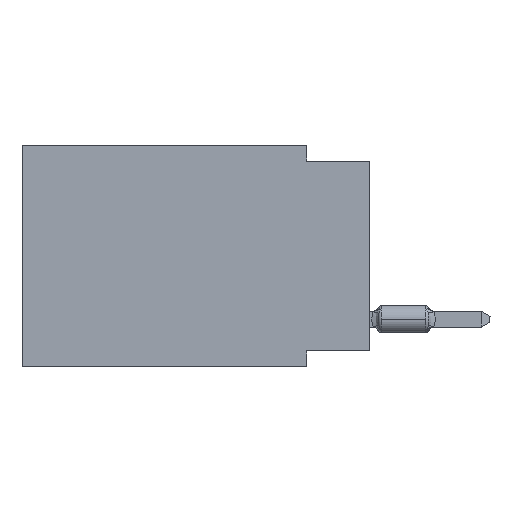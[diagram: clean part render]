
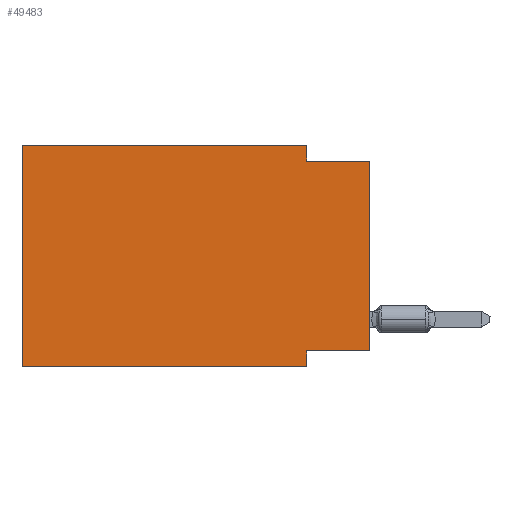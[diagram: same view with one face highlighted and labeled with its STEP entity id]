
A CAD part, left-side view. The second image highlights one B-rep face of the part: STEP entity #49483.
In plain terms, the highlighted planar face has unit normal (-1, 0, 0).
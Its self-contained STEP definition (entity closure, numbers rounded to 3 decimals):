
#1197 = CARTESIAN_POINT ( 'NONE',  ( 0., 2.54, -0.635 ) ) ;
#2183 = LINE ( 'NONE', #63998, #44489 ) ;
#3015 = VERTEX_POINT ( 'NONE', #1197 ) ;
#3428 = CARTESIAN_POINT ( 'NONE',  ( 0., 0., 0. ) ) ;
#4145 = EDGE_CURVE ( 'NONE', #8017, #71424, #2183, .T. ) ;
#4315 = LINE ( 'NONE', #15302, #61417 ) ;
#7125 = ORIENTED_EDGE ( 'NONE', *, *, #34295, .F. ) ;
#7843 = EDGE_CURVE ( 'NONE', #71424, #58549, #4315, .T. ) ;
#8017 = VERTEX_POINT ( 'NONE', #29485 ) ;
#8047 = DIRECTION ( 'NONE',  ( 0., 1., 0. ) ) ;
#8056 = AXIS2_PLACEMENT_3D ( 'NONE', #58355, #60075, #41530 ) ;
#8127 = ORIENTED_EDGE ( 'NONE', *, *, #29234, .F. ) ;
#9586 = EDGE_LOOP ( 'NONE', ( #41284, #8127, #21846, #18374, #7125, #32060, #51661, #27058 ) ) ;
#9642 = EDGE_CURVE ( 'NONE', #36503, #58549, #62520, .T. ) ;
#11381 = CARTESIAN_POINT ( 'NONE',  ( 0., 13.97, -8.89 ) ) ;
#13303 = CARTESIAN_POINT ( 'NONE',  ( 0., 2.54, -8.255 ) ) ;
#15302 = CARTESIAN_POINT ( 'NONE',  ( 0., 2.54, -8.89 ) ) ;
#16020 = VECTOR ( 'NONE', #38916, 1000. ) ;
#17001 = LINE ( 'NONE', #29404, #69201 ) ;
#17892 = CARTESIAN_POINT ( 'NONE',  ( 0., 2.54, 0. ) ) ;
#18254 = DIRECTION ( 'NONE',  ( 0., -1., 0. ) ) ;
#18374 = ORIENTED_EDGE ( 'NONE', *, *, #44616, .F. ) ;
#21582 = CARTESIAN_POINT ( 'NONE',  ( 0., 2.54, -8.89 ) ) ;
#21825 = CARTESIAN_POINT ( 'NONE',  ( 0., 13.97, 0. ) ) ;
#21846 = ORIENTED_EDGE ( 'NONE', *, *, #62630, .F. ) ;
#21873 = DIRECTION ( 'NONE',  ( 0., 0., -1. ) ) ;
#23708 = VERTEX_POINT ( 'NONE', #62487 ) ;
#27058 = ORIENTED_EDGE ( 'NONE', *, *, #4145, .F. ) ;
#27232 = CARTESIAN_POINT ( 'NONE',  ( 0., 0., -0.635 ) ) ;
#29214 = CARTESIAN_POINT ( 'NONE',  ( 0., 13.97, -8.89 ) ) ;
#29234 = EDGE_CURVE ( 'NONE', #3015, #56450, #61934, .T. ) ;
#29404 = CARTESIAN_POINT ( 'NONE',  ( 0., 13.97, 0. ) ) ;
#29485 = CARTESIAN_POINT ( 'NONE',  ( 0., 0., -8.255 ) ) ;
#32060 = ORIENTED_EDGE ( 'NONE', *, *, #9642, .T. ) ;
#32788 = LINE ( 'NONE', #21825, #62432 ) ;
#34295 = EDGE_CURVE ( 'NONE', #36503, #23708, #32788, .T. ) ;
#36503 = VERTEX_POINT ( 'NONE', #11381 ) ;
#37451 = DIRECTION ( 'NONE',  ( 0., 0., 1. ) ) ;
#38234 = VECTOR ( 'NONE', #18254, 1000. ) ;
#38916 = DIRECTION ( 'NONE',  ( 0., -1., 0. ) ) ;
#39303 = DIRECTION ( 'NONE',  ( 0., -1., 0. ) ) ;
#41284 = ORIENTED_EDGE ( 'NONE', *, *, #41306, .T. ) ;
#41306 = EDGE_CURVE ( 'NONE', #8017, #56450, #58668, .T. ) ;
#41530 = DIRECTION ( 'NONE',  ( 0., 0., -1. ) ) ;
#44489 = VECTOR ( 'NONE', #8047, 1000. ) ;
#44616 = EDGE_CURVE ( 'NONE', #23708, #46604, #17001, .T. ) ;
#46604 = VERTEX_POINT ( 'NONE', #17892 ) ;
#48545 = DIRECTION ( 'NONE',  ( 0., 0., 1. ) ) ;
#49483 = ADVANCED_FACE ( 'NONE', ( #52505 ), #71057, .F. ) ;
#49727 = CARTESIAN_POINT ( 'NONE',  ( 0., 2.54, 0. ) ) ;
#51661 = ORIENTED_EDGE ( 'NONE', *, *, #7843, .F. ) ;
#52091 = VECTOR ( 'NONE', #72384, 1000. ) ;
#52505 = FACE_OUTER_BOUND ( 'NONE', #9586, .T. ) ;
#56272 = LINE ( 'NONE', #49727, #52091 ) ;
#56450 = VERTEX_POINT ( 'NONE', #66959 ) ;
#58355 = CARTESIAN_POINT ( 'NONE',  ( 0., 13.97, 0. ) ) ;
#58549 = VERTEX_POINT ( 'NONE', #21582 ) ;
#58668 = LINE ( 'NONE', #3428, #66522 ) ;
#60075 = DIRECTION ( 'NONE',  ( 1., 0., 0. ) ) ;
#61417 = VECTOR ( 'NONE', #21873, 1000. ) ;
#61934 = LINE ( 'NONE', #27232, #16020 ) ;
#62432 = VECTOR ( 'NONE', #48545, 1000. ) ;
#62487 = CARTESIAN_POINT ( 'NONE',  ( 0., 13.97, 0. ) ) ;
#62520 = LINE ( 'NONE', #29214, #38234 ) ;
#62630 = EDGE_CURVE ( 'NONE', #46604, #3015, #56272, .T. ) ;
#63998 = CARTESIAN_POINT ( 'NONE',  ( 0., 0., -8.255 ) ) ;
#66522 = VECTOR ( 'NONE', #37451, 1000. ) ;
#66959 = CARTESIAN_POINT ( 'NONE',  ( 0., 0., -0.635 ) ) ;
#69201 = VECTOR ( 'NONE', #39303, 1000. ) ;
#71057 = PLANE ( 'NONE',  #8056 ) ;
#71424 = VERTEX_POINT ( 'NONE', #13303 ) ;
#72384 = DIRECTION ( 'NONE',  ( 0., 0., -1. ) ) ;
